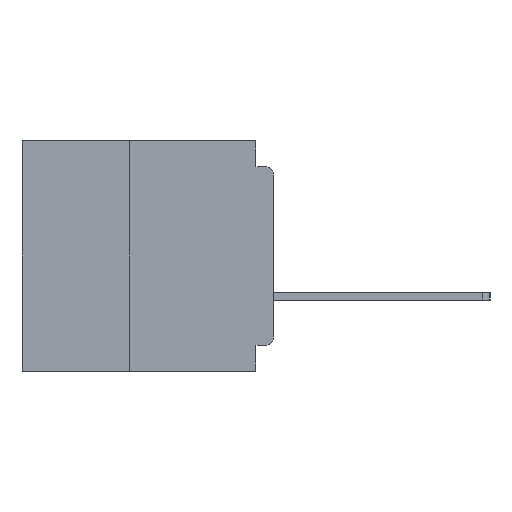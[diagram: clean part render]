
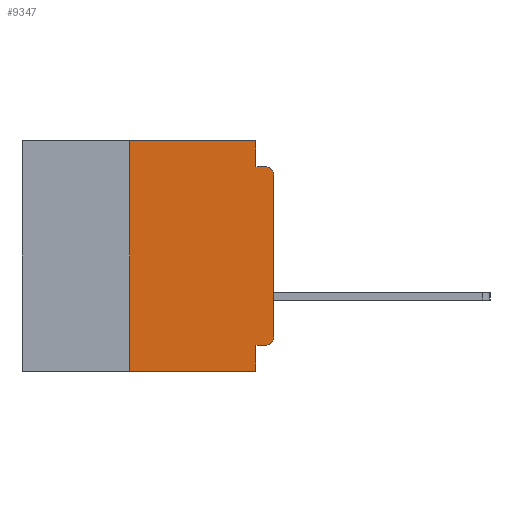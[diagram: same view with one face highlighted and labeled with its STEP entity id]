
A CAD part, left-side view. The second image highlights one B-rep face of the part: STEP entity #9347.
In plain terms, the highlighted planar face has unit normal (-1, 0, 0).
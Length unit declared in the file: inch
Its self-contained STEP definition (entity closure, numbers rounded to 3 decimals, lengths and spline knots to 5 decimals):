
#398 = EDGE_CURVE ( 'NONE', #28158, #19673, #9876, .T. ) ;
#746 = CARTESIAN_POINT ( 'NONE',  ( 0., 0.25, -0.4 ) ) ;
#1724 = VERTEX_POINT ( 'NONE', #41580 ) ;
#2172 = PLANE ( 'NONE',  #38372 ) ;
#4942 = CARTESIAN_POINT ( 'NONE',  ( 0., 0.25, 0. ) ) ;
#5045 = CARTESIAN_POINT ( 'NONE',  ( 0., 0.015, -0.355 ) ) ;
#5845 = EDGE_CURVE ( 'NONE', #7063, #42587, #40854, .T. ) ;
#5942 = DIRECTION ( 'NONE',  ( 0., 0., -1. ) ) ;
#6227 = CARTESIAN_POINT ( 'NONE',  ( 0., 0.031, -0.045 ) ) ;
#6337 = ORIENTED_EDGE ( 'NONE', *, *, #398, .F. ) ;
#7063 = VERTEX_POINT ( 'NONE', #746 ) ;
#7344 = EDGE_CURVE ( 'NONE', #1724, #10773, #33438, .T. ) ;
#8120 = EDGE_CURVE ( 'NONE', #19673, #28364, #28293, .T. ) ;
#8766 = CARTESIAN_POINT ( 'NONE',  ( 0., 0., -0.045 ) ) ;
#8954 = DIRECTION ( 'NONE',  ( 0., 0., -1. ) ) ;
#9089 = DIRECTION ( 'NONE',  ( 0., 0., 1. ) ) ;
#9347 = ADVANCED_FACE ( 'NONE', ( #25322 ), #2172, .F. ) ;
#9876 = LINE ( 'NONE', #19233, #19791 ) ;
#10773 = VERTEX_POINT ( 'NONE', #14998 ) ;
#13259 = DIRECTION ( 'NONE',  ( 0., 1., 0. ) ) ;
#13904 = CARTESIAN_POINT ( 'NONE',  ( 0., 0.031, 0. ) ) ;
#13911 = VECTOR ( 'NONE', #9089, 39.37008 ) ;
#14998 = CARTESIAN_POINT ( 'NONE',  ( 0., 0., -0.06 ) ) ;
#15344 = CARTESIAN_POINT ( 'NONE',  ( 0., 0.031, -0.4 ) ) ;
#15392 = ORIENTED_EDGE ( 'NONE', *, *, #38389, .T. ) ;
#16304 = CARTESIAN_POINT ( 'NONE',  ( 0., 0.031, -0.355 ) ) ;
#16810 = CARTESIAN_POINT ( 'NONE',  ( 0., 0., -0.355 ) ) ;
#17038 = CARTESIAN_POINT ( 'NONE',  ( 0., 0.437, 0. ) ) ;
#17092 = VECTOR ( 'NONE', #21854, 39.37008 ) ;
#17318 = VECTOR ( 'NONE', #25096, 39.37008 ) ;
#18129 = CARTESIAN_POINT ( 'NONE',  ( 0., 0.25, -0.4 ) ) ;
#18137 = CARTESIAN_POINT ( 'NONE',  ( 0., 0.015, -0.06 ) ) ;
#19233 = CARTESIAN_POINT ( 'NONE',  ( 0., 0.437, 0. ) ) ;
#19245 = ORIENTED_EDGE ( 'NONE', *, *, #8120, .F. ) ;
#19319 = DIRECTION ( 'NONE',  ( -1., 0., 0. ) ) ;
#19454 = LINE ( 'NONE', #18129, #17092 ) ;
#19673 = VERTEX_POINT ( 'NONE', #33930 ) ;
#19765 = VERTEX_POINT ( 'NONE', #16304 ) ;
#19791 = VECTOR ( 'NONE', #21435, 39.37008 ) ;
#21409 = DIRECTION ( 'NONE',  ( 0., -1., 0. ) ) ;
#21435 = DIRECTION ( 'NONE',  ( 0., -1., 0. ) ) ;
#21854 = DIRECTION ( 'NONE',  ( 0., 0., 1. ) ) ;
#21859 = DIRECTION ( 'NONE',  ( 0., 0., -1. ) ) ;
#22458 = AXIS2_PLACEMENT_3D ( 'NONE', #41100, #19319, #44715 ) ;
#23105 = CARTESIAN_POINT ( 'NONE',  ( 0., 0.437, -0.4 ) ) ;
#23605 = DIRECTION ( 'NONE',  ( 0., -1., 0. ) ) ;
#23927 = CIRCLE ( 'NONE', #43313, 0.015 ) ;
#24065 = EDGE_CURVE ( 'NONE', #28773, #19765, #46164, .T. ) ;
#25096 = DIRECTION ( 'NONE',  ( 0., 0., -1. ) ) ;
#25322 = FACE_OUTER_BOUND ( 'NONE', #32077, .T. ) ;
#25360 = ORIENTED_EDGE ( 'NONE', *, *, #24065, .F. ) ;
#26827 = VECTOR ( 'NONE', #8954, 39.37008 ) ;
#27485 = EDGE_CURVE ( 'NONE', #28364, #30079, #44544, .T. ) ;
#28158 = VERTEX_POINT ( 'NONE', #4942 ) ;
#28185 = DIRECTION ( 'NONE',  ( 1., 0., 0. ) ) ;
#28293 = LINE ( 'NONE', #13904, #17318 ) ;
#28364 = VERTEX_POINT ( 'NONE', #6227 ) ;
#28456 = EDGE_CURVE ( 'NONE', #7063, #28158, #19454, .T. ) ;
#28773 = VERTEX_POINT ( 'NONE', #5045 ) ;
#29388 = CARTESIAN_POINT ( 'NONE',  ( 0., 0.015, -0.045 ) ) ;
#30031 = EDGE_CURVE ( 'NONE', #10773, #30079, #23927, .T. ) ;
#30079 = VERTEX_POINT ( 'NONE', #29388 ) ;
#30132 = VECTOR ( 'NONE', #21409, 39.37008 ) ;
#31945 = ORIENTED_EDGE ( 'NONE', *, *, #7344, .T. ) ;
#32077 = EDGE_LOOP ( 'NONE', ( #31945, #40454, #35142, #19245, #6337, #42360, #38441, #35910, #25360, #15392 ) ) ;
#33438 = LINE ( 'NONE', #38437, #13911 ) ;
#33930 = CARTESIAN_POINT ( 'NONE',  ( 0., 0.031, 0. ) ) ;
#34926 = VECTOR ( 'NONE', #23605, 39.37008 ) ;
#35142 = ORIENTED_EDGE ( 'NONE', *, *, #27485, .F. ) ;
#35910 = ORIENTED_EDGE ( 'NONE', *, *, #46708, .F. ) ;
#36407 = LINE ( 'NONE', #38155, #26827 ) ;
#38155 = CARTESIAN_POINT ( 'NONE',  ( 0., 0.031, -0.4 ) ) ;
#38372 = AXIS2_PLACEMENT_3D ( 'NONE', #17038, #28185, #5942 ) ;
#38389 = EDGE_CURVE ( 'NONE', #28773, #1724, #44162, .T. ) ;
#38437 = CARTESIAN_POINT ( 'NONE',  ( 0., 0., 0. ) ) ;
#38441 = ORIENTED_EDGE ( 'NONE', *, *, #5845, .T. ) ;
#40454 = ORIENTED_EDGE ( 'NONE', *, *, #30031, .T. ) ;
#40854 = LINE ( 'NONE', #23105, #30132 ) ;
#41100 = CARTESIAN_POINT ( 'NONE',  ( 0., 0.015, -0.34 ) ) ;
#41580 = CARTESIAN_POINT ( 'NONE',  ( 0., 0., -0.34 ) ) ;
#42360 = ORIENTED_EDGE ( 'NONE', *, *, #28456, .F. ) ;
#42587 = VERTEX_POINT ( 'NONE', #15344 ) ;
#43313 = AXIS2_PLACEMENT_3D ( 'NONE', #18137, #43585, #21859 ) ;
#43585 = DIRECTION ( 'NONE',  ( -1., 0., 0. ) ) ;
#44162 = CIRCLE ( 'NONE', #22458, 0.015 ) ;
#44544 = LINE ( 'NONE', #8766, #34926 ) ;
#44715 = DIRECTION ( 'NONE',  ( 0., 0., -1. ) ) ;
#45051 = VECTOR ( 'NONE', #13259, 39.37008 ) ;
#46164 = LINE ( 'NONE', #16810, #45051 ) ;
#46708 = EDGE_CURVE ( 'NONE', #19765, #42587, #36407, .T. ) ;
